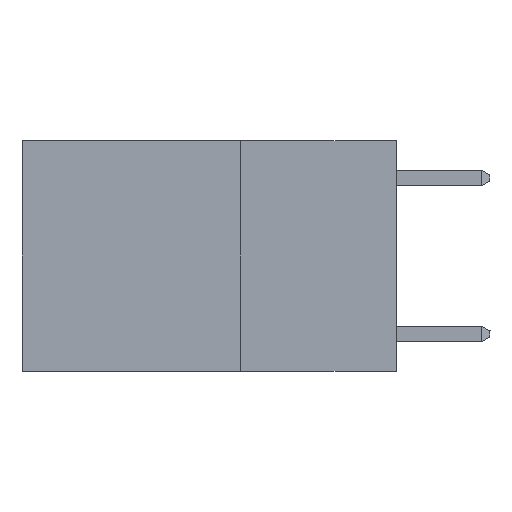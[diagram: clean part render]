
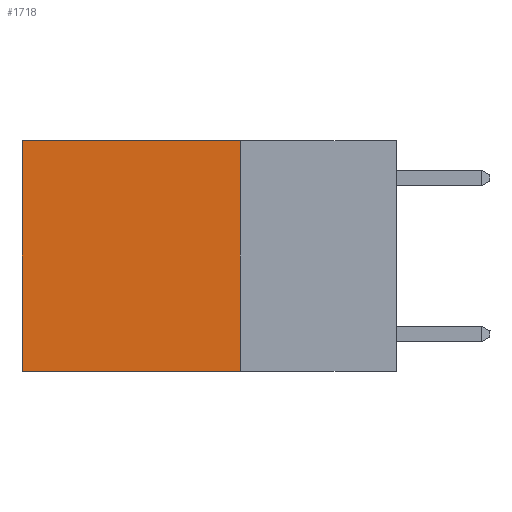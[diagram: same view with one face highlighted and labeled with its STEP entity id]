
A CAD part, left-side view. The second image highlights one B-rep face of the part: STEP entity #1718.
In plain terms, the highlighted planar face has unit normal (-1, 0, 0).
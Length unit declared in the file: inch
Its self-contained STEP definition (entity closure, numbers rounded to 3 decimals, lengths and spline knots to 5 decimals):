
#677 = EDGE_CURVE ( 'NONE', #3887, #11732, #11068, .T. ) ;
#979 = VECTOR ( 'NONE', #17304, 39.37008 ) ;
#1241 = EDGE_CURVE ( 'NONE', #12919, #12176, #15801, .T. ) ;
#1506 = CARTESIAN_POINT ( 'NONE',  ( 0.2625, 0.25, 0. ) ) ;
#1643 = CARTESIAN_POINT ( 'NONE',  ( 0.2625, 0.6, 0. ) ) ;
#1718 = ADVANCED_FACE ( 'NONE', ( #10531 ), #10438, .F. ) ;
#2587 = DIRECTION ( 'NONE',  ( 0., 1., 0. ) ) ;
#2926 = ORIENTED_EDGE ( 'NONE', *, *, #8702, .F. ) ;
#3887 = VERTEX_POINT ( 'NONE', #11611 ) ;
#5167 = VECTOR ( 'NONE', #2587, 39.37008 ) ;
#5715 = CARTESIAN_POINT ( 'NONE',  ( 0.2625, 0.6, 0. ) ) ;
#6318 = LINE ( 'NONE', #16314, #5167 ) ;
#6974 = VECTOR ( 'NONE', #9494, 39.37008 ) ;
#8297 = AXIS2_PLACEMENT_3D ( 'NONE', #1506, #8968, #13558 ) ;
#8386 = CARTESIAN_POINT ( 'NONE',  ( 0.2625, 0.25, -0.37 ) ) ;
#8396 = CARTESIAN_POINT ( 'NONE',  ( 0.2625, 0.6, -0.37 ) ) ;
#8702 = EDGE_CURVE ( 'NONE', #11732, #12176, #16890, .T. ) ;
#8968 = DIRECTION ( 'NONE',  ( 1., 0., 0. ) ) ;
#9494 = DIRECTION ( 'NONE',  ( 0., 0., -1. ) ) ;
#10025 = EDGE_CURVE ( 'NONE', #3887, #12919, #6318, .T. ) ;
#10438 = PLANE ( 'NONE',  #8297 ) ;
#10531 = FACE_OUTER_BOUND ( 'NONE', #13905, .T. ) ;
#10689 = DIRECTION ( 'NONE',  ( 0., 0., -1. ) ) ;
#11068 = LINE ( 'NONE', #15474, #6974 ) ;
#11611 = CARTESIAN_POINT ( 'NONE',  ( 0.2625, 0.25, 0. ) ) ;
#11732 = VERTEX_POINT ( 'NONE', #16280 ) ;
#12176 = VERTEX_POINT ( 'NONE', #8396 ) ;
#12919 = VERTEX_POINT ( 'NONE', #5715 ) ;
#13558 = DIRECTION ( 'NONE',  ( 0., 0., -1. ) ) ;
#13905 = EDGE_LOOP ( 'NONE', ( #15351, #2926, #16583, #14539 ) ) ;
#14539 = ORIENTED_EDGE ( 'NONE', *, *, #10025, .T. ) ;
#15351 = ORIENTED_EDGE ( 'NONE', *, *, #1241, .T. ) ;
#15474 = CARTESIAN_POINT ( 'NONE',  ( 0.2625, 0.25, 0. ) ) ;
#15801 = LINE ( 'NONE', #1643, #19608 ) ;
#16280 = CARTESIAN_POINT ( 'NONE',  ( 0.2625, 0.25, -0.37 ) ) ;
#16314 = CARTESIAN_POINT ( 'NONE',  ( 0.2625, 0.25, 0. ) ) ;
#16583 = ORIENTED_EDGE ( 'NONE', *, *, #677, .F. ) ;
#16890 = LINE ( 'NONE', #8386, #979 ) ;
#17304 = DIRECTION ( 'NONE',  ( 0., 1., 0. ) ) ;
#19608 = VECTOR ( 'NONE', #10689, 39.37008 ) ;
